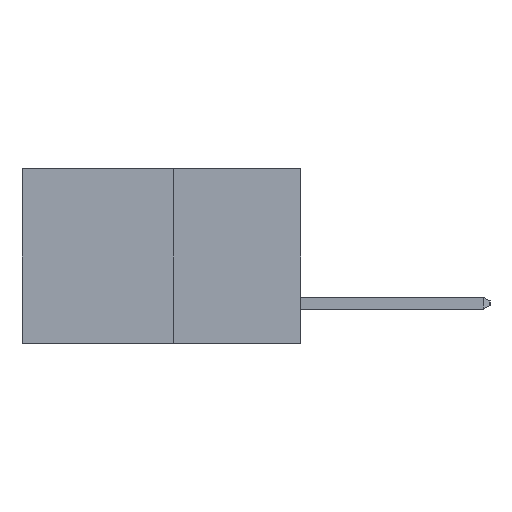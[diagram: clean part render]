
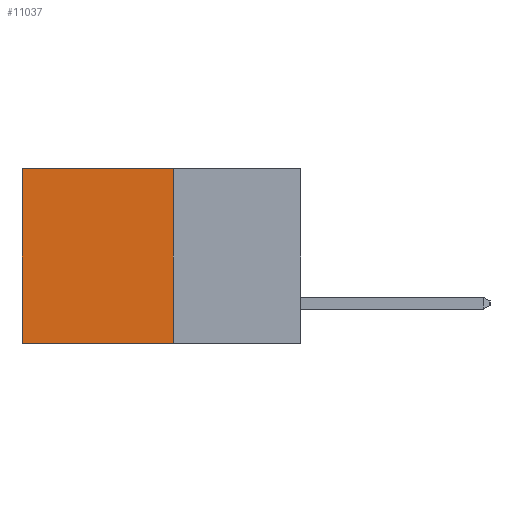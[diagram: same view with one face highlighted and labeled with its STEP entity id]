
A CAD part, left-side view. The second image highlights one B-rep face of the part: STEP entity #11037.
In plain terms, the highlighted planar face has unit normal (-1, 0, 0).
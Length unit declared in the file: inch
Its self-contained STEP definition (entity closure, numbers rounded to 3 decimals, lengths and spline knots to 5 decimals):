
#327 = LINE ( 'NONE', #2351, #2863 ) ;
#878 = PLANE ( 'NONE',  #9109 ) ;
#1953 = DIRECTION ( 'NONE',  ( 1., 0., 0. ) ) ;
#2351 = CARTESIAN_POINT ( 'NONE',  ( 0.277, 0.27, -0.37 ) ) ;
#2863 = VECTOR ( 'NONE', #12973, 39.37008 ) ;
#3229 = CARTESIAN_POINT ( 'NONE',  ( 0.277, 0.59, 0. ) ) ;
#4889 = VERTEX_POINT ( 'NONE', #6690 ) ;
#5239 = ORIENTED_EDGE ( 'NONE', *, *, #12403, .T. ) ;
#5265 = CARTESIAN_POINT ( 'NONE',  ( 0.277, 0.27, -0.37 ) ) ;
#5510 = VECTOR ( 'NONE', #8409, 39.37008 ) ;
#5614 = VECTOR ( 'NONE', #7435, 39.37008 ) ;
#6090 = DIRECTION ( 'NONE',  ( 0., 0., -1. ) ) ;
#6110 = LINE ( 'NONE', #10287, #13513 ) ;
#6690 = CARTESIAN_POINT ( 'NONE',  ( 0.277, 0.59, -0.37 ) ) ;
#7132 = VERTEX_POINT ( 'NONE', #3229 ) ;
#7435 = DIRECTION ( 'NONE',  ( 0., 0., -1. ) ) ;
#7753 = VERTEX_POINT ( 'NONE', #5265 ) ;
#8303 = EDGE_CURVE ( 'NONE', #7132, #4889, #6110, .T. ) ;
#8381 = CARTESIAN_POINT ( 'NONE',  ( 0.277, 0.27, -0.37 ) ) ;
#8409 = DIRECTION ( 'NONE',  ( 0., 1., 0. ) ) ;
#8484 = EDGE_CURVE ( 'NONE', #11042, #7753, #13669, .T. ) ;
#9109 = AXIS2_PLACEMENT_3D ( 'NONE', #8381, #1953, #9434 ) ;
#9434 = DIRECTION ( 'NONE',  ( 0., 0., -1. ) ) ;
#10287 = CARTESIAN_POINT ( 'NONE',  ( 0.277, 0.59, -0.37 ) ) ;
#10475 = CARTESIAN_POINT ( 'NONE',  ( 0.277, 0.27, 0. ) ) ;
#10504 = ORIENTED_EDGE ( 'NONE', *, *, #10645, .F. ) ;
#10645 = EDGE_CURVE ( 'NONE', #7753, #4889, #327, .T. ) ;
#10679 = ORIENTED_EDGE ( 'NONE', *, *, #8484, .F. ) ;
#10721 = EDGE_LOOP ( 'NONE', ( #12966, #10504, #10679, #5239 ) ) ;
#11037 = ADVANCED_FACE ( 'NONE', ( #12303 ), #878, .F. ) ;
#11042 = VERTEX_POINT ( 'NONE', #10475 ) ;
#11479 = LINE ( 'NONE', #13611, #5510 ) ;
#12303 = FACE_OUTER_BOUND ( 'NONE', #10721, .T. ) ;
#12403 = EDGE_CURVE ( 'NONE', #11042, #7132, #11479, .T. ) ;
#12966 = ORIENTED_EDGE ( 'NONE', *, *, #8303, .T. ) ;
#12973 = DIRECTION ( 'NONE',  ( 0., 1., 0. ) ) ;
#13513 = VECTOR ( 'NONE', #6090, 39.37008 ) ;
#13611 = CARTESIAN_POINT ( 'NONE',  ( 0.277, 0.27, 0. ) ) ;
#13669 = LINE ( 'NONE', #13714, #5614 ) ;
#13714 = CARTESIAN_POINT ( 'NONE',  ( 0.277, 0.27, -0.37 ) ) ;
